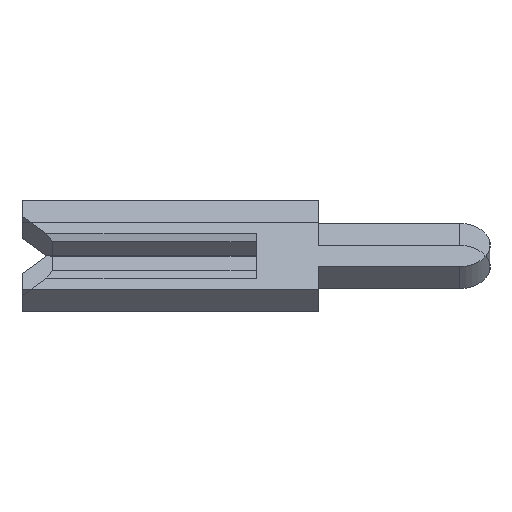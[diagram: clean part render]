
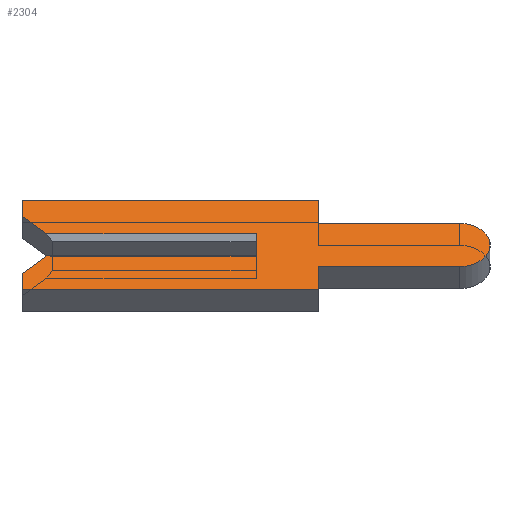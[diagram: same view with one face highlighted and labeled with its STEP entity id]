
A CAD part, left-side view. The second image highlights one B-rep face of the part: STEP entity #2304.
In plain terms, the highlighted face is planar.
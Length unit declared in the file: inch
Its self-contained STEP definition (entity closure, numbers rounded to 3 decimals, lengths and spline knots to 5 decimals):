
#76 = CARTESIAN_POINT ( 'NONE',  ( -0.01, -0.1305, 0.0195 ) ) ;
#85 = ORIENTED_EDGE ( 'NONE', *, *, #1687, .T. ) ;
#87 = CARTESIAN_POINT ( 'NONE',  ( -0.01, 0.15, 0.026 ) ) ;
#98 = EDGE_CURVE ( 'NONE', #1691, #1441, #183, .T. ) ;
#110 = FACE_OUTER_BOUND ( 'NONE', #979, .T. ) ;
#124 = CARTESIAN_POINT ( 'NONE',  ( -0.01, -0.04, -0.0195 ) ) ;
#134 = VECTOR ( 'NONE', #2438, 39.37008 ) ;
#149 = ORIENTED_EDGE ( 'NONE', *, *, #1879, .F. ) ;
#169 = CARTESIAN_POINT ( 'NONE',  ( -0.01, 0.134, 0.01 ) ) ;
#183 = LINE ( 'NONE', #1856, #663 ) ;
#193 = ORIENTED_EDGE ( 'NONE', *, *, #560, .F. ) ;
#205 = DIRECTION ( 'NONE',  ( 1., 0., 0. ) ) ;
#239 = EDGE_CURVE ( 'NONE', #500, #897, #639, .T. ) ;
#260 = EDGE_CURVE ( 'NONE', #1990, #1691, #1975, .T. ) ;
#262 = VECTOR ( 'NONE', #2502, 39.37008 ) ;
#317 = EDGE_CURVE ( 'NONE', #1662, #620, #2070, .T. ) ;
#356 = ORIENTED_EDGE ( 'NONE', *, *, #1611, .F. ) ;
#381 = VERTEX_POINT ( 'NONE', #1457 ) ;
#410 = LINE ( 'NONE', #1046, #1958 ) ;
#416 = ORIENTED_EDGE ( 'NONE', *, *, #98, .F. ) ;
#438 = CARTESIAN_POINT ( 'NONE',  ( -0.01, -0.04, 0.04 ) ) ;
#445 = VERTEX_POINT ( 'NONE', #2083 ) ;
#468 = LINE ( 'NONE', #1646, #1093 ) ;
#476 = LINE ( 'NONE', #1833, #134 ) ;
#488 = ORIENTED_EDGE ( 'NONE', *, *, #1315, .F. ) ;
#500 = VERTEX_POINT ( 'NONE', #855 ) ;
#513 = CARTESIAN_POINT ( 'NONE',  ( -0.01, 0.1305, 0.0065 ) ) ;
#560 = EDGE_CURVE ( 'NONE', #2328, #2129, #1070, .T. ) ;
#605 = CARTESIAN_POINT ( 'NONE',  ( -0.01, 0.15, -0.026 ) ) ;
#620 = VERTEX_POINT ( 'NONE', #1138 ) ;
#637 = CARTESIAN_POINT ( 'NONE',  ( -0.01, -0.04, -0.0195 ) ) ;
#639 = LINE ( 'NONE', #2274, #1587 ) ;
#648 = DIRECTION ( 'NONE',  ( 0., 0., 1. ) ) ;
#663 = VECTOR ( 'NONE', #1702, 39.37008 ) ;
#682 = CARTESIAN_POINT ( 'NONE',  ( -0.01, -0.1305, -0.0195 ) ) ;
#855 = CARTESIAN_POINT ( 'NONE',  ( -0.01, 0., -0.01 ) ) ;
#867 = LINE ( 'NONE', #513, #262 ) ;
#870 = DIRECTION ( 'NONE',  ( 0., 0., 1. ) ) ;
#881 = DIRECTION ( 'NONE',  ( 0., 0., -1. ) ) ;
#897 = VERTEX_POINT ( 'NONE', #1976 ) ;
#912 = EDGE_CURVE ( 'NONE', #381, #1662, #1998, .T. ) ;
#940 = VERTEX_POINT ( 'NONE', #169 ) ;
#963 = ORIENTED_EDGE ( 'NONE', *, *, #1863, .F. ) ;
#967 = AXIS2_PLACEMENT_3D ( 'NONE', #2401, #205, #995 ) ;
#978 = LINE ( 'NONE', #2228, #2387 ) ;
#979 = EDGE_LOOP ( 'NONE', ( #85, #2201, #356, #2293, #1301, #963, #416, #2512, #488, #193, #1033, #2436, #149, #2485 ) ) ;
#995 = DIRECTION ( 'NONE',  ( 0., 0., -1. ) ) ;
#1033 = ORIENTED_EDGE ( 'NONE', *, *, #2011, .F. ) ;
#1039 = DIRECTION ( 'NONE',  ( 0., -0.707, 0.707 ) ) ;
#1040 = VECTOR ( 'NONE', #1039, 39.37008 ) ;
#1046 = CARTESIAN_POINT ( 'NONE',  ( -0.01, -0.04, 0.04 ) ) ;
#1070 = LINE ( 'NONE', #1564, #1559 ) ;
#1078 = PLANE ( 'NONE',  #1770 ) ;
#1093 = VECTOR ( 'NONE', #1419, 39.37008 ) ;
#1111 = DIRECTION ( 'NONE',  ( 0., 1., 0. ) ) ;
#1138 = CARTESIAN_POINT ( 'NONE',  ( -0.01, 0.134, -0.01 ) ) ;
#1202 = LINE ( 'NONE', #2426, #2282 ) ;
#1261 = CIRCLE ( 'NONE', #967, 0.0195 ) ;
#1289 = CARTESIAN_POINT ( 'NONE',  ( -0.01, -0.1305, 0. ) ) ;
#1295 = VECTOR ( 'NONE', #1111, 39.37008 ) ;
#1301 = ORIENTED_EDGE ( 'NONE', *, *, #912, .F. ) ;
#1314 = DIRECTION ( 'NONE',  ( 0., 0., 1. ) ) ;
#1315 = EDGE_CURVE ( 'NONE', #2129, #1990, #1261, .T. ) ;
#1419 = DIRECTION ( 'NONE',  ( 0., -1., 0. ) ) ;
#1429 = CARTESIAN_POINT ( 'NONE',  ( -0.01, -0.04, -0.04 ) ) ;
#1441 = VERTEX_POINT ( 'NONE', #1429 ) ;
#1450 = VECTOR ( 'NONE', #1314, 39.37008 ) ;
#1457 = CARTESIAN_POINT ( 'NONE',  ( -0.01, 0.15, -0.04 ) ) ;
#1477 = VECTOR ( 'NONE', #870, 39.37008 ) ;
#1490 = CARTESIAN_POINT ( 'NONE',  ( -0.01, 0.15, 0.026 ) ) ;
#1519 = CARTESIAN_POINT ( 'NONE',  ( -0.01, 0.1305, -0.0065 ) ) ;
#1543 = CARTESIAN_POINT ( 'NONE',  ( -0.01, 0.15, -0.026 ) ) ;
#1559 = VECTOR ( 'NONE', #1738, 39.37008 ) ;
#1564 = CARTESIAN_POINT ( 'NONE',  ( -0.01, -0.04, 0.0195 ) ) ;
#1587 = VECTOR ( 'NONE', #648, 39.37008 ) ;
#1611 = EDGE_CURVE ( 'NONE', #620, #500, #468, .T. ) ;
#1646 = CARTESIAN_POINT ( 'NONE',  ( -0.01, -0.1305, -0.01 ) ) ;
#1662 = VERTEX_POINT ( 'NONE', #605 ) ;
#1687 = EDGE_CURVE ( 'NONE', #940, #897, #1202, .T. ) ;
#1691 = VERTEX_POINT ( 'NONE', #637 ) ;
#1693 = DIRECTION ( 'NONE',  ( 0., 0., -1. ) ) ;
#1702 = DIRECTION ( 'NONE',  ( 0., 0., -1. ) ) ;
#1707 = DIRECTION ( 'NONE',  ( 1., 0., 0. ) ) ;
#1714 = CARTESIAN_POINT ( 'NONE',  ( -0.01, -0.04, 0.0195 ) ) ;
#1738 = DIRECTION ( 'NONE',  ( 0., -1., 0. ) ) ;
#1751 = VERTEX_POINT ( 'NONE', #438 ) ;
#1770 = AXIS2_PLACEMENT_3D ( 'NONE', #1289, #1707, #1693 ) ;
#1803 = DIRECTION ( 'NONE',  ( 0., 1., 0. ) ) ;
#1821 = EDGE_CURVE ( 'NONE', #445, #1751, #476, .T. ) ;
#1833 = CARTESIAN_POINT ( 'NONE',  ( -0.01, 0.15, 0.04 ) ) ;
#1856 = CARTESIAN_POINT ( 'NONE',  ( -0.01, -0.04, -0.04 ) ) ;
#1863 = EDGE_CURVE ( 'NONE', #1441, #381, #978, .T. ) ;
#1879 = EDGE_CURVE ( 'NONE', #1987, #445, #2325, .T. ) ;
#1958 = VECTOR ( 'NONE', #881, 39.37008 ) ;
#1975 = LINE ( 'NONE', #124, #1295 ) ;
#1976 = CARTESIAN_POINT ( 'NONE',  ( -0.01, 0., 0.01 ) ) ;
#1987 = VERTEX_POINT ( 'NONE', #87 ) ;
#1990 = VERTEX_POINT ( 'NONE', #682 ) ;
#1998 = LINE ( 'NONE', #1543, #1450 ) ;
#2011 = EDGE_CURVE ( 'NONE', #1751, #2328, #410, .T. ) ;
#2041 = DIRECTION ( 'NONE',  ( 0., -1., 0. ) ) ;
#2070 = LINE ( 'NONE', #1519, #1040 ) ;
#2083 = CARTESIAN_POINT ( 'NONE',  ( -0.01, 0.15, 0.04 ) ) ;
#2129 = VERTEX_POINT ( 'NONE', #76 ) ;
#2201 = ORIENTED_EDGE ( 'NONE', *, *, #239, .F. ) ;
#2228 = CARTESIAN_POINT ( 'NONE',  ( -0.01, 0.15, -0.04 ) ) ;
#2274 = CARTESIAN_POINT ( 'NONE',  ( -0.01, 0., 0.0065 ) ) ;
#2282 = VECTOR ( 'NONE', #2041, 39.37008 ) ;
#2293 = ORIENTED_EDGE ( 'NONE', *, *, #317, .F. ) ;
#2304 = ADVANCED_FACE ( 'NONE', ( #110 ), #1078, .F. ) ;
#2325 = LINE ( 'NONE', #1490, #1477 ) ;
#2328 = VERTEX_POINT ( 'NONE', #1714 ) ;
#2387 = VECTOR ( 'NONE', #1803, 39.37008 ) ;
#2401 = CARTESIAN_POINT ( 'NONE',  ( -0.01, -0.1305, 0. ) ) ;
#2426 = CARTESIAN_POINT ( 'NONE',  ( -0.01, 0.15, 0.01 ) ) ;
#2436 = ORIENTED_EDGE ( 'NONE', *, *, #1821, .F. ) ;
#2438 = DIRECTION ( 'NONE',  ( 0., -1., 0. ) ) ;
#2485 = ORIENTED_EDGE ( 'NONE', *, *, #2526, .F. ) ;
#2502 = DIRECTION ( 'NONE',  ( 0., 0.707, 0.707 ) ) ;
#2512 = ORIENTED_EDGE ( 'NONE', *, *, #260, .F. ) ;
#2526 = EDGE_CURVE ( 'NONE', #940, #1987, #867, .T. ) ;
